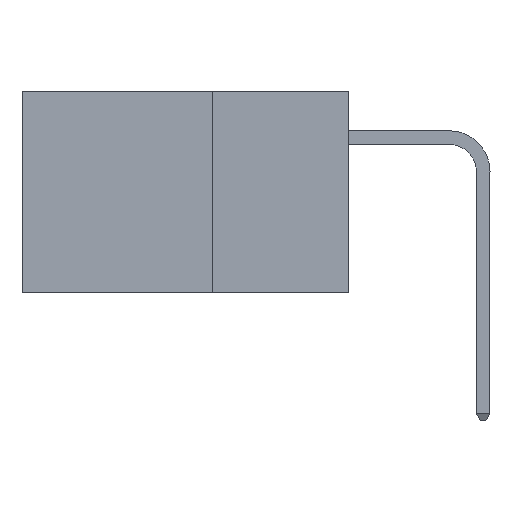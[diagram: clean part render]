
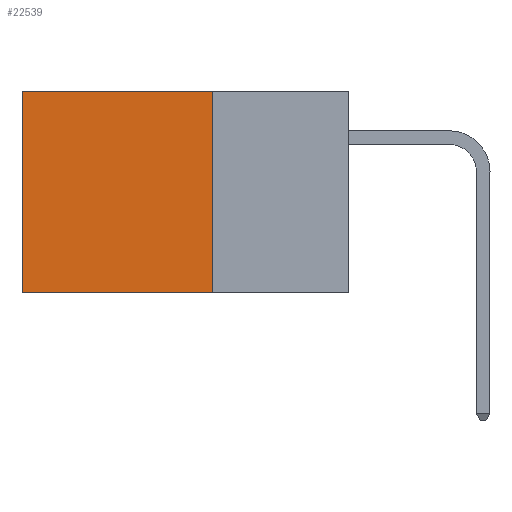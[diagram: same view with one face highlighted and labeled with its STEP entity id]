
A CAD part, left-side view. The second image highlights one B-rep face of the part: STEP entity #22539.
In plain terms, the highlighted planar face has unit normal (-1, 0, 0).
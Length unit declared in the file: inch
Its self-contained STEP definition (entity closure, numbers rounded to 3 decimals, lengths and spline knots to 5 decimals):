
#759 = CARTESIAN_POINT ( 'NONE',  ( 0.2875, 0.25, 0. ) ) ;
#2597 = CARTESIAN_POINT ( 'NONE',  ( 0.2875, 0.6, 0. ) ) ;
#3322 = CARTESIAN_POINT ( 'NONE',  ( 0.2875, 0.25, 0. ) ) ;
#3481 = VERTEX_POINT ( 'NONE', #2597 ) ;
#4836 = PLANE ( 'NONE',  #7974 ) ;
#5359 = DIRECTION ( 'NONE',  ( 0., 1., 0. ) ) ;
#5374 = LINE ( 'NONE', #3322, #26103 ) ;
#6859 = DIRECTION ( 'NONE',  ( 0., 0., -1. ) ) ;
#7501 = ORIENTED_EDGE ( 'NONE', *, *, #20753, .F. ) ;
#7974 = AXIS2_PLACEMENT_3D ( 'NONE', #759, #18913, #6859 ) ;
#8589 = VERTEX_POINT ( 'NONE', #17372 ) ;
#11378 = LINE ( 'NONE', #21407, #11989 ) ;
#11631 = LINE ( 'NONE', #16465, #18208 ) ;
#11989 = VECTOR ( 'NONE', #15209, 39.37008 ) ;
#12120 = CARTESIAN_POINT ( 'NONE',  ( 0.2875, 0.6, -0.37 ) ) ;
#12131 = VERTEX_POINT ( 'NONE', #12120 ) ;
#12553 = DIRECTION ( 'NONE',  ( 0., 0., -1. ) ) ;
#14009 = ORIENTED_EDGE ( 'NONE', *, *, #14719, .T. ) ;
#14060 = FACE_OUTER_BOUND ( 'NONE', #15589, .T. ) ;
#14719 = EDGE_CURVE ( 'NONE', #3481, #12131, #16095, .T. ) ;
#15209 = DIRECTION ( 'NONE',  ( 0., 0., -1. ) ) ;
#15589 = EDGE_LOOP ( 'NONE', ( #14009, #19278, #7501, #25474 ) ) ;
#16095 = LINE ( 'NONE', #22573, #18005 ) ;
#16465 = CARTESIAN_POINT ( 'NONE',  ( 0.2875, 0.25, -0.37 ) ) ;
#16604 = EDGE_CURVE ( 'NONE', #22176, #12131, #11631, .T. ) ;
#17372 = CARTESIAN_POINT ( 'NONE',  ( 0.2875, 0.25, 0. ) ) ;
#18005 = VECTOR ( 'NONE', #12553, 39.37008 ) ;
#18208 = VECTOR ( 'NONE', #20572, 39.37008 ) ;
#18913 = DIRECTION ( 'NONE',  ( 1., 0., 0. ) ) ;
#19278 = ORIENTED_EDGE ( 'NONE', *, *, #16604, .F. ) ;
#19945 = CARTESIAN_POINT ( 'NONE',  ( 0.2875, 0.25, -0.37 ) ) ;
#20572 = DIRECTION ( 'NONE',  ( 0., 1., 0. ) ) ;
#20753 = EDGE_CURVE ( 'NONE', #8589, #22176, #11378, .T. ) ;
#20781 = EDGE_CURVE ( 'NONE', #8589, #3481, #5374, .T. ) ;
#21407 = CARTESIAN_POINT ( 'NONE',  ( 0.2875, 0.25, 0. ) ) ;
#22176 = VERTEX_POINT ( 'NONE', #19945 ) ;
#22539 = ADVANCED_FACE ( 'NONE', ( #14060 ), #4836, .F. ) ;
#22573 = CARTESIAN_POINT ( 'NONE',  ( 0.2875, 0.6, 0. ) ) ;
#25474 = ORIENTED_EDGE ( 'NONE', *, *, #20781, .T. ) ;
#26103 = VECTOR ( 'NONE', #5359, 39.37008 ) ;
